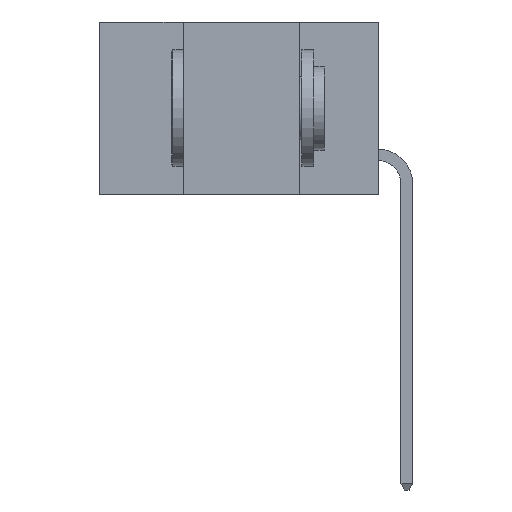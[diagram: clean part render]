
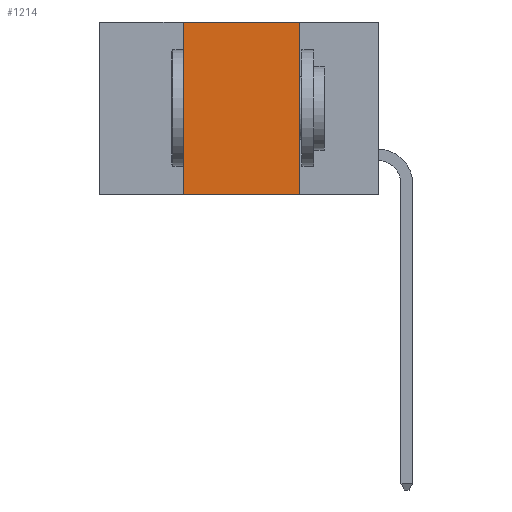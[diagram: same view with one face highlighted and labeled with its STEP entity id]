
A CAD part, left-side view. The second image highlights one B-rep face of the part: STEP entity #1214.
In plain terms, the highlighted planar face has unit normal (-1, 0, 0).
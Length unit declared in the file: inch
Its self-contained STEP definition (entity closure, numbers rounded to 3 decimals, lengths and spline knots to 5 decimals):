
#218 = DIRECTION ( 'NONE',  ( 0., -1., 0. ) ) ;
#1162 = ORIENTED_EDGE ( 'NONE', *, *, #6569, .T. ) ;
#1214 = ADVANCED_FACE ( 'NONE', ( #5698 ), #7028, .F. ) ;
#1399 = CARTESIAN_POINT ( 'NONE',  ( 0., 0.6, 0. ) ) ;
#3035 = ORIENTED_EDGE ( 'NONE', *, *, #6438, .F. ) ;
#3261 = DIRECTION ( 'NONE',  ( 0., 0., -1. ) ) ;
#3383 = CARTESIAN_POINT ( 'NONE',  ( 0., 0.42, -0.37 ) ) ;
#3572 = VERTEX_POINT ( 'NONE', #5879 ) ;
#3605 = ORIENTED_EDGE ( 'NONE', *, *, #12084, .F. ) ;
#4033 = VECTOR ( 'NONE', #7711, 39.37008 ) ;
#5028 = VERTEX_POINT ( 'NONE', #3383 ) ;
#5597 = CARTESIAN_POINT ( 'NONE',  ( 0., 0.6, 0. ) ) ;
#5698 = FACE_OUTER_BOUND ( 'NONE', #14368, .T. ) ;
#5879 = CARTESIAN_POINT ( 'NONE',  ( 0., 0.17, 0. ) ) ;
#6023 = AXIS2_PLACEMENT_3D ( 'NONE', #5597, #18272, #3261 ) ;
#6438 = EDGE_CURVE ( 'NONE', #3572, #10351, #15943, .T. ) ;
#6466 = VECTOR ( 'NONE', #10083, 39.37008 ) ;
#6569 = EDGE_CURVE ( 'NONE', #5028, #10351, #9929, .T. ) ;
#7028 = PLANE ( 'NONE',  #6023 ) ;
#7702 = EDGE_CURVE ( 'NONE', #5028, #14504, #7761, .T. ) ;
#7711 = DIRECTION ( 'NONE',  ( 0., -1., 0. ) ) ;
#7761 = LINE ( 'NONE', #14864, #16663 ) ;
#8002 = CARTESIAN_POINT ( 'NONE',  ( 0., 0.42, 0. ) ) ;
#8281 = CARTESIAN_POINT ( 'NONE',  ( 0., 0.6, -0.37 ) ) ;
#9717 = CARTESIAN_POINT ( 'NONE',  ( 0., 0.17, -0.37 ) ) ;
#9929 = LINE ( 'NONE', #8281, #4033 ) ;
#10083 = DIRECTION ( 'NONE',  ( 0., 0., -1. ) ) ;
#10351 = VERTEX_POINT ( 'NONE', #10646 ) ;
#10646 = CARTESIAN_POINT ( 'NONE',  ( 0., 0.17, -0.37 ) ) ;
#12084 = EDGE_CURVE ( 'NONE', #14504, #3572, #17146, .T. ) ;
#12739 = VECTOR ( 'NONE', #218, 39.37008 ) ;
#14368 = EDGE_LOOP ( 'NONE', ( #3035, #3605, #18126, #1162 ) ) ;
#14504 = VERTEX_POINT ( 'NONE', #8002 ) ;
#14765 = DIRECTION ( 'NONE',  ( 0., 0., 1. ) ) ;
#14864 = CARTESIAN_POINT ( 'NONE',  ( 0., 0.42, -0.37 ) ) ;
#15943 = LINE ( 'NONE', #9717, #6466 ) ;
#16663 = VECTOR ( 'NONE', #14765, 39.37008 ) ;
#17146 = LINE ( 'NONE', #1399, #12739 ) ;
#18126 = ORIENTED_EDGE ( 'NONE', *, *, #7702, .F. ) ;
#18272 = DIRECTION ( 'NONE',  ( 1., 0., 0. ) ) ;
